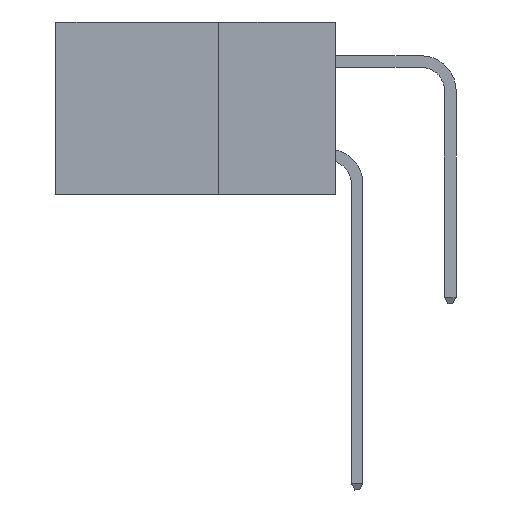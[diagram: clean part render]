
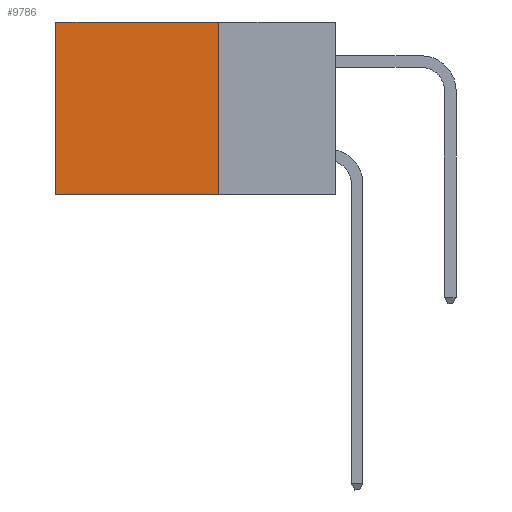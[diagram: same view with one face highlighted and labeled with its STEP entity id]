
A CAD part, left-side view. The second image highlights one B-rep face of the part: STEP entity #9786.
In plain terms, the highlighted planar face has unit normal (-1, 0, 0).
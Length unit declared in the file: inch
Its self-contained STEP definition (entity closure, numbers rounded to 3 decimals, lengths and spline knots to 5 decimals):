
#1635 = FACE_OUTER_BOUND ( 'NONE', #16254, .T. ) ;
#2806 = CARTESIAN_POINT ( 'NONE',  ( 0.2875, 0.25, -0.37 ) ) ;
#3592 = EDGE_CURVE ( 'NONE', #25336, #23495, #6608, .T. ) ;
#3914 = DIRECTION ( 'NONE',  ( 1., 0., 0. ) ) ;
#5065 = DIRECTION ( 'NONE',  ( 0., 1., 0. ) ) ;
#5572 = VERTEX_POINT ( 'NONE', #18715 ) ;
#6608 = LINE ( 'NONE', #22392, #23688 ) ;
#8678 = PLANE ( 'NONE',  #13367 ) ;
#9786 = ADVANCED_FACE ( 'NONE', ( #1635 ), #8678, .F. ) ;
#10010 = ORIENTED_EDGE ( 'NONE', *, *, #15256, .F. ) ;
#11980 = ORIENTED_EDGE ( 'NONE', *, *, #20044, .T. ) ;
#12639 = VECTOR ( 'NONE', #19695, 39.37008 ) ;
#13367 = AXIS2_PLACEMENT_3D ( 'NONE', #15033, #3914, #19515 ) ;
#13900 = LINE ( 'NONE', #25563, #22306 ) ;
#15033 = CARTESIAN_POINT ( 'NONE',  ( 0.2875, 0.25, 0. ) ) ;
#15256 = EDGE_CURVE ( 'NONE', #25336, #15627, #13900, .T. ) ;
#15627 = VERTEX_POINT ( 'NONE', #27996 ) ;
#15766 = ORIENTED_EDGE ( 'NONE', *, *, #3592, .T. ) ;
#16254 = EDGE_LOOP ( 'NONE', ( #11980, #27008, #10010, #15766 ) ) ;
#17449 = CARTESIAN_POINT ( 'NONE',  ( 0.2875, 0.6, 0. ) ) ;
#18715 = CARTESIAN_POINT ( 'NONE',  ( 0.2875, 0.6, -0.37 ) ) ;
#19515 = DIRECTION ( 'NONE',  ( 0., 0., -1. ) ) ;
#19695 = DIRECTION ( 'NONE',  ( 0., 0., -1. ) ) ;
#20044 = EDGE_CURVE ( 'NONE', #23495, #5572, #23133, .T. ) ;
#20162 = DIRECTION ( 'NONE',  ( 0., 0., -1. ) ) ;
#20437 = VECTOR ( 'NONE', #5065, 39.37008 ) ;
#22306 = VECTOR ( 'NONE', #20162, 39.37008 ) ;
#22392 = CARTESIAN_POINT ( 'NONE',  ( 0.2875, 0.25, 0. ) ) ;
#23133 = LINE ( 'NONE', #17449, #12639 ) ;
#23495 = VERTEX_POINT ( 'NONE', #24128 ) ;
#23688 = VECTOR ( 'NONE', #24626, 39.37008 ) ;
#24128 = CARTESIAN_POINT ( 'NONE',  ( 0.2875, 0.6, 0. ) ) ;
#24626 = DIRECTION ( 'NONE',  ( 0., 1., 0. ) ) ;
#25336 = VERTEX_POINT ( 'NONE', #25494 ) ;
#25373 = EDGE_CURVE ( 'NONE', #15627, #5572, #26408, .T. ) ;
#25494 = CARTESIAN_POINT ( 'NONE',  ( 0.2875, 0.25, 0. ) ) ;
#25563 = CARTESIAN_POINT ( 'NONE',  ( 0.2875, 0.25, 0. ) ) ;
#26408 = LINE ( 'NONE', #2806, #20437 ) ;
#27008 = ORIENTED_EDGE ( 'NONE', *, *, #25373, .F. ) ;
#27996 = CARTESIAN_POINT ( 'NONE',  ( 0.2875, 0.25, -0.37 ) ) ;
